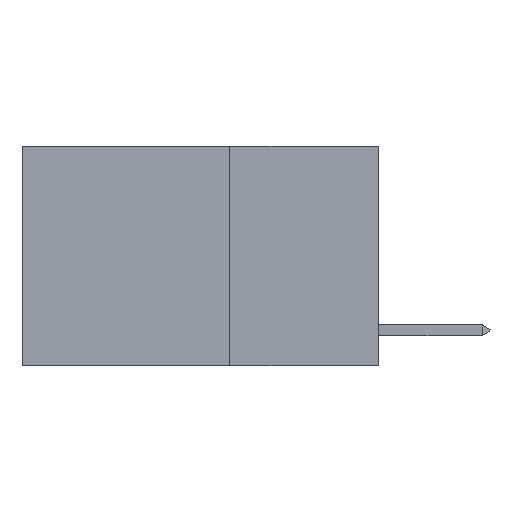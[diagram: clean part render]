
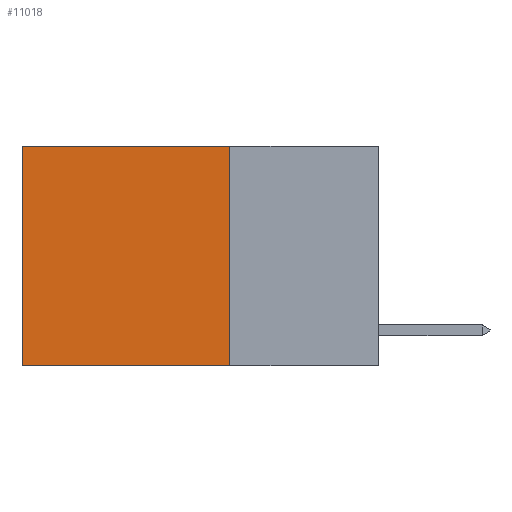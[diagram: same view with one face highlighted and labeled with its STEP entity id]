
A CAD part, left-side view. The second image highlights one B-rep face of the part: STEP entity #11018.
In plain terms, the highlighted planar face has unit normal (-1, 0, 0).
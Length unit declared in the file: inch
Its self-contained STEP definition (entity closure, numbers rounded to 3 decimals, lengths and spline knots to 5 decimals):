
#563 = DIRECTION ( 'NONE',  ( 0., 0., -1. ) ) ;
#567 = EDGE_CURVE ( 'NONE', #6585, #5106, #4532, .T. ) ;
#1334 = LINE ( 'NONE', #16405, #11184 ) ;
#1951 = VERTEX_POINT ( 'NONE', #17632 ) ;
#3145 = ORIENTED_EDGE ( 'NONE', *, *, #12902, .T. ) ;
#3777 = PLANE ( 'NONE',  #9986 ) ;
#4299 = ORIENTED_EDGE ( 'NONE', *, *, #11740, .F. ) ;
#4308 = DIRECTION ( 'NONE',  ( 0., 1., 0. ) ) ;
#4532 = LINE ( 'NONE', #4652, #20698 ) ;
#4544 = EDGE_LOOP ( 'NONE', ( #12799, #4299, #6604, #3145 ) ) ;
#4639 = CARTESIAN_POINT ( 'NONE',  ( 0.2625, 0.25, -0.37 ) ) ;
#4652 = CARTESIAN_POINT ( 'NONE',  ( 0.2625, 0.6, 0. ) ) ;
#5106 = VERTEX_POINT ( 'NONE', #11623 ) ;
#5849 = LINE ( 'NONE', #4639, #7397 ) ;
#5962 = VERTEX_POINT ( 'NONE', #18904 ) ;
#6585 = VERTEX_POINT ( 'NONE', #17705 ) ;
#6604 = ORIENTED_EDGE ( 'NONE', *, *, #15714, .F. ) ;
#7397 = VECTOR ( 'NONE', #11225, 39.37008 ) ;
#9481 = DIRECTION ( 'NONE',  ( 0., 0., -1. ) ) ;
#9986 = AXIS2_PLACEMENT_3D ( 'NONE', #19280, #10721, #17201 ) ;
#10459 = LINE ( 'NONE', #12220, #14079 ) ;
#10721 = DIRECTION ( 'NONE',  ( 1., 0., 0. ) ) ;
#11018 = ADVANCED_FACE ( 'NONE', ( #12473 ), #3777, .F. ) ;
#11184 = VECTOR ( 'NONE', #4308, 39.37008 ) ;
#11225 = DIRECTION ( 'NONE',  ( 0., 1., 0. ) ) ;
#11623 = CARTESIAN_POINT ( 'NONE',  ( 0.2625, 0.6, -0.37 ) ) ;
#11740 = EDGE_CURVE ( 'NONE', #1951, #5106, #5849, .T. ) ;
#12220 = CARTESIAN_POINT ( 'NONE',  ( 0.2625, 0.25, 0. ) ) ;
#12473 = FACE_OUTER_BOUND ( 'NONE', #4544, .T. ) ;
#12799 = ORIENTED_EDGE ( 'NONE', *, *, #567, .T. ) ;
#12902 = EDGE_CURVE ( 'NONE', #5962, #6585, #1334, .T. ) ;
#14079 = VECTOR ( 'NONE', #563, 39.37008 ) ;
#15714 = EDGE_CURVE ( 'NONE', #5962, #1951, #10459, .T. ) ;
#16405 = CARTESIAN_POINT ( 'NONE',  ( 0.2625, 0.25, 0. ) ) ;
#17201 = DIRECTION ( 'NONE',  ( 0., 0., -1. ) ) ;
#17632 = CARTESIAN_POINT ( 'NONE',  ( 0.2625, 0.25, -0.37 ) ) ;
#17705 = CARTESIAN_POINT ( 'NONE',  ( 0.2625, 0.6, 0. ) ) ;
#18904 = CARTESIAN_POINT ( 'NONE',  ( 0.2625, 0.25, 0. ) ) ;
#19280 = CARTESIAN_POINT ( 'NONE',  ( 0.2625, 0.25, 0. ) ) ;
#20698 = VECTOR ( 'NONE', #9481, 39.37008 ) ;
